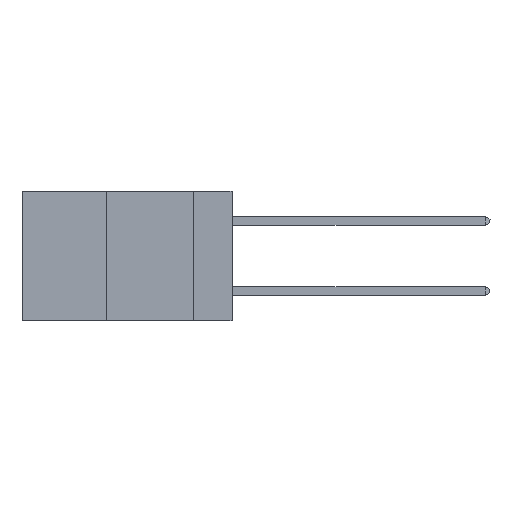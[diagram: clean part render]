
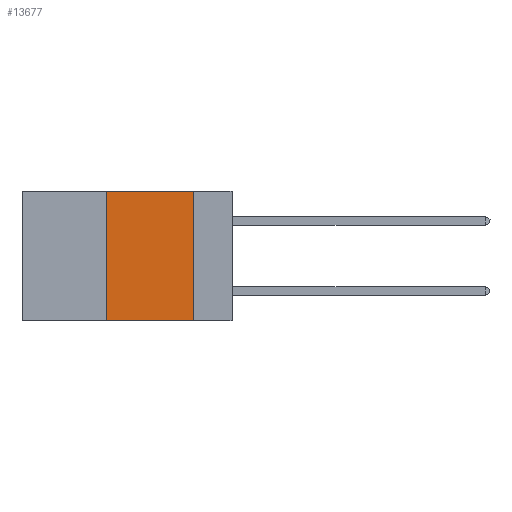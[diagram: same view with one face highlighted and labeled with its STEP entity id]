
A CAD part, left-side view. The second image highlights one B-rep face of the part: STEP entity #13677.
In plain terms, the highlighted planar face has unit normal (-1, 0, 0).
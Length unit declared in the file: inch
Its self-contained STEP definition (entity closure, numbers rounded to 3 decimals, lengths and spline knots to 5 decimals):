
#629 = ORIENTED_EDGE ( 'NONE', *, *, #32955, .T. ) ;
#1062 = EDGE_CURVE ( 'NONE', #37631, #37573, #31316, .T. ) ;
#1530 = CARTESIAN_POINT ( 'NONE',  ( 0., 0.6, 0. ) ) ;
#2113 = EDGE_CURVE ( 'NONE', #30085, #37631, #13610, .T. ) ;
#2233 = EDGE_LOOP ( 'NONE', ( #11384, #40888, #32110, #629 ) ) ;
#4446 = DIRECTION ( 'NONE',  ( 0., -1., 0. ) ) ;
#5031 = LINE ( 'NONE', #27955, #23296 ) ;
#7560 = CARTESIAN_POINT ( 'NONE',  ( 0., 0.11, 0. ) ) ;
#9505 = VECTOR ( 'NONE', #4446, 39.37008 ) ;
#11384 = ORIENTED_EDGE ( 'NONE', *, *, #1062, .F. ) ;
#12138 = DIRECTION ( 'NONE',  ( 0., 0., -1. ) ) ;
#12263 = DIRECTION ( 'NONE',  ( 0., 0., -1. ) ) ;
#13610 = LINE ( 'NONE', #1530, #9505 ) ;
#13677 = ADVANCED_FACE ( 'NONE', ( #40603 ), #31441, .F. ) ;
#14641 = CARTESIAN_POINT ( 'NONE',  ( 0., 0.36, 0. ) ) ;
#15455 = LINE ( 'NONE', #31500, #17841 ) ;
#16077 = DIRECTION ( 'NONE',  ( 0., -1., 0. ) ) ;
#17469 = CARTESIAN_POINT ( 'NONE',  ( 0., 0.36, -0.37 ) ) ;
#17841 = VECTOR ( 'NONE', #16077, 39.37008 ) ;
#18362 = DIRECTION ( 'NONE',  ( 0., 0., 1. ) ) ;
#20448 = EDGE_CURVE ( 'NONE', #26644, #30085, #5031, .T. ) ;
#21639 = DIRECTION ( 'NONE',  ( 1., 0., 0. ) ) ;
#23296 = VECTOR ( 'NONE', #18362, 39.37008 ) ;
#26534 = AXIS2_PLACEMENT_3D ( 'NONE', #34144, #21639, #12263 ) ;
#26628 = VECTOR ( 'NONE', #12138, 39.37008 ) ;
#26644 = VERTEX_POINT ( 'NONE', #17469 ) ;
#27955 = CARTESIAN_POINT ( 'NONE',  ( 0., 0.36, 0. ) ) ;
#30085 = VERTEX_POINT ( 'NONE', #14641 ) ;
#31316 = LINE ( 'NONE', #34827, #26628 ) ;
#31441 = PLANE ( 'NONE',  #26534 ) ;
#31500 = CARTESIAN_POINT ( 'NONE',  ( 0., 0.6, -0.37 ) ) ;
#32110 = ORIENTED_EDGE ( 'NONE', *, *, #20448, .F. ) ;
#32157 = CARTESIAN_POINT ( 'NONE',  ( 0., 0.11, -0.37 ) ) ;
#32955 = EDGE_CURVE ( 'NONE', #26644, #37573, #15455, .T. ) ;
#34144 = CARTESIAN_POINT ( 'NONE',  ( 0., 0.6, 0. ) ) ;
#34827 = CARTESIAN_POINT ( 'NONE',  ( 0., 0.11, 0. ) ) ;
#37573 = VERTEX_POINT ( 'NONE', #32157 ) ;
#37631 = VERTEX_POINT ( 'NONE', #7560 ) ;
#40603 = FACE_OUTER_BOUND ( 'NONE', #2233, .T. ) ;
#40888 = ORIENTED_EDGE ( 'NONE', *, *, #2113, .F. ) ;
